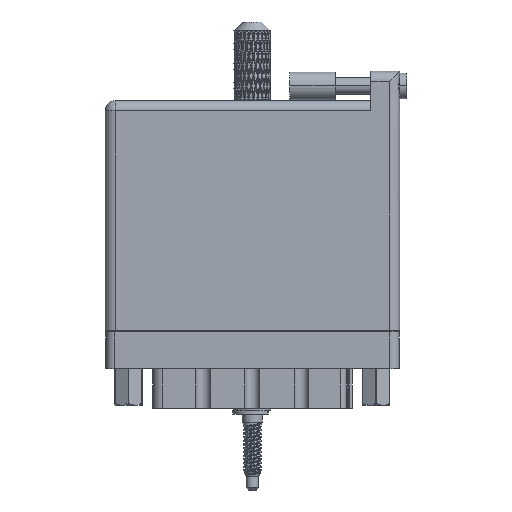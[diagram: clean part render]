
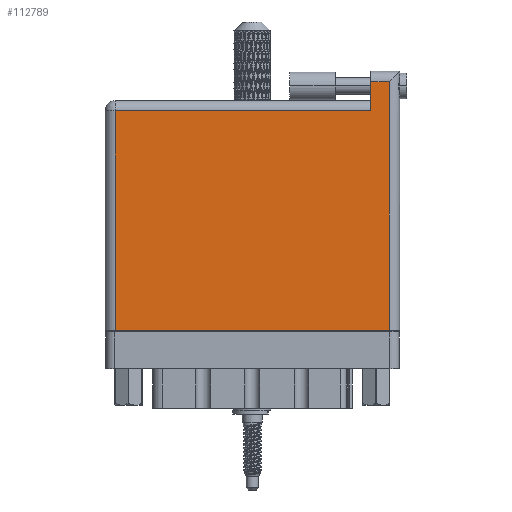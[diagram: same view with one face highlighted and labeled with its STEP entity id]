
A CAD part, front view. The second image highlights one B-rep face of the part: STEP entity #112789.
In plain terms, the highlighted face is planar.
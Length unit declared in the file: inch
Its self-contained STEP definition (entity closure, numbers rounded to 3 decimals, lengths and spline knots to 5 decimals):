
#4170 = EDGE_CURVE ( 'NONE', #108418, #30056, #41652, .T. ) ;
#7863 = CARTESIAN_POINT ( 'NONE',  ( 1.938, 1.766, 0. ) ) ;
#12210 = DIRECTION ( 'NONE',  ( -1., 0., 0. ) ) ;
#15511 = ORIENTED_EDGE ( 'NONE', *, *, #55162, .T. ) ;
#21285 = VECTOR ( 'NONE', #97759, 39.37008 ) ;
#23910 = CARTESIAN_POINT ( 'NONE',  ( 1.811, 1.696, 0. ) ) ;
#24124 = AXIS2_PLACEMENT_3D ( 'NONE', #46813, #46417, #12210 ) ;
#24155 = VERTEX_POINT ( 'NONE', #103512 ) ;
#30056 = VERTEX_POINT ( 'NONE', #56192 ) ;
#34659 = VECTOR ( 'NONE', #102114, 39.37008 ) ;
#35165 = ORIENTED_EDGE ( 'NONE', *, *, #91780, .T. ) ;
#39731 = FACE_OUTER_BOUND ( 'NONE', #58058, .T. ) ;
#41652 = LINE ( 'NONE', #67495, #44458 ) ;
#42937 = CARTESIAN_POINT ( 'NONE',  ( 0., 0., 0. ) ) ;
#44458 = VECTOR ( 'NONE', #110323, 39.37008 ) ;
#45788 = LINE ( 'NONE', #93138, #34659 ) ;
#46417 = DIRECTION ( 'NONE',  ( 0., 0., -1. ) ) ;
#46767 = VERTEX_POINT ( 'NONE', #23910 ) ;
#46813 = CARTESIAN_POINT ( 'NONE',  ( 0., 1.566, 0. ) ) ;
#47010 = CARTESIAN_POINT ( 'NONE',  ( 1.811, 1.766, 0. ) ) ;
#53419 = DIRECTION ( 'NONE',  ( -1., 0., 0. ) ) ;
#55107 = EDGE_CURVE ( 'NONE', #86537, #24155, #67639, .T. ) ;
#55162 = EDGE_CURVE ( 'NONE', #62939, #46767, #65477, .T. ) ;
#55237 = VECTOR ( 'NONE', #73434, 39.37008 ) ;
#55734 = CARTESIAN_POINT ( 'NONE',  ( 1.811, 1.496, 0. ) ) ;
#56192 = CARTESIAN_POINT ( 'NONE',  ( 0.07, 1.496, 0. ) ) ;
#56556 = PLANE ( 'NONE',  #24124 ) ;
#58058 = EDGE_LOOP ( 'NONE', ( #94388, #35165, #15511, #103636, #67509, #109920 ) ) ;
#58074 = LINE ( 'NONE', #47010, #55237 ) ;
#62008 = VECTOR ( 'NONE', #113805, 39.37008 ) ;
#62939 = VERTEX_POINT ( 'NONE', #108520 ) ;
#65477 = LINE ( 'NONE', #88060, #86344 ) ;
#67495 = CARTESIAN_POINT ( 'NONE',  ( 0., 1.496, 0. ) ) ;
#67509 = ORIENTED_EDGE ( 'NONE', *, *, #4170, .T. ) ;
#67639 = LINE ( 'NONE', #42937, #62008 ) ;
#73434 = DIRECTION ( 'NONE',  ( 0., -1., 0. ) ) ;
#76112 = EDGE_CURVE ( 'NONE', #46767, #108418, #58074, .T. ) ;
#86147 = EDGE_CURVE ( 'NONE', #30056, #86537, #45788, .T. ) ;
#86344 = VECTOR ( 'NONE', #53419, 39.37008 ) ;
#86537 = VERTEX_POINT ( 'NONE', #101590 ) ;
#88060 = CARTESIAN_POINT ( 'NONE',  ( 0., 1.696, 0. ) ) ;
#91780 = EDGE_CURVE ( 'NONE', #24155, #62939, #104826, .T. ) ;
#93138 = CARTESIAN_POINT ( 'NONE',  ( 0.07, 0., 0. ) ) ;
#94388 = ORIENTED_EDGE ( 'NONE', *, *, #55107, .T. ) ;
#97759 = DIRECTION ( 'NONE',  ( 0., 1., 0. ) ) ;
#101590 = CARTESIAN_POINT ( 'NONE',  ( 0.07, 0., 0. ) ) ;
#102114 = DIRECTION ( 'NONE',  ( 0., -1., 0. ) ) ;
#103512 = CARTESIAN_POINT ( 'NONE',  ( 1.938, 0., 0. ) ) ;
#103636 = ORIENTED_EDGE ( 'NONE', *, *, #76112, .T. ) ;
#104826 = LINE ( 'NONE', #7863, #21285 ) ;
#108418 = VERTEX_POINT ( 'NONE', #55734 ) ;
#108520 = CARTESIAN_POINT ( 'NONE',  ( 1.938, 1.696, 0. ) ) ;
#109920 = ORIENTED_EDGE ( 'NONE', *, *, #86147, .T. ) ;
#110323 = DIRECTION ( 'NONE',  ( -1., 0., 0. ) ) ;
#112789 = ADVANCED_FACE ( 'NONE', ( #39731 ), #56556, .F. ) ;
#113805 = DIRECTION ( 'NONE',  ( 1., 0., 0. ) ) ;
